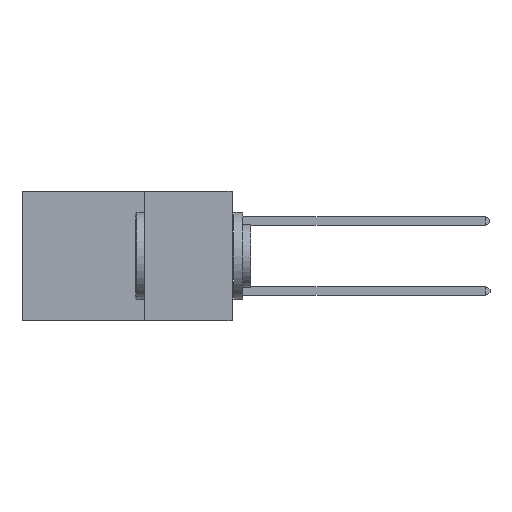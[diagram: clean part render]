
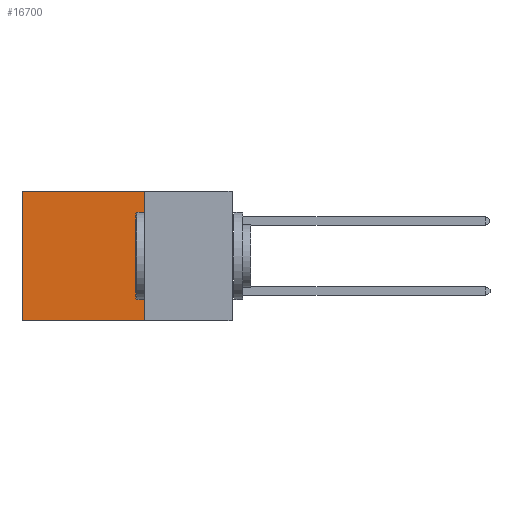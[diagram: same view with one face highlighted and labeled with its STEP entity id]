
A CAD part, left-side view. The second image highlights one B-rep face of the part: STEP entity #16700.
In plain terms, the highlighted planar face has unit normal (-1, 0, 0).
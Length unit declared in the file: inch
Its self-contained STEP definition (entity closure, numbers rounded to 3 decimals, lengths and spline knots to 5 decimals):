
#1242 = ORIENTED_EDGE ( 'NONE', *, *, #16120, .F. ) ;
#1254 = VECTOR ( 'NONE', #3936, 39.37008 ) ;
#3865 = VERTEX_POINT ( 'NONE', #8342 ) ;
#3936 = DIRECTION ( 'NONE',  ( 0., 0., -1. ) ) ;
#3940 = VERTEX_POINT ( 'NONE', #5247 ) ;
#5247 = CARTESIAN_POINT ( 'NONE',  ( 0.2875, 0.6, -0.37 ) ) ;
#5428 = LINE ( 'NONE', #10939, #1254 ) ;
#6461 = PLANE ( 'NONE',  #10349 ) ;
#6723 = CARTESIAN_POINT ( 'NONE',  ( 0.2875, 0.25, 0. ) ) ;
#7794 = EDGE_CURVE ( 'NONE', #13338, #8580, #21814, .T. ) ;
#8181 = DIRECTION ( 'NONE',  ( 0., 1., 0. ) ) ;
#8248 = DIRECTION ( 'NONE',  ( 0., 0., -1. ) ) ;
#8342 = CARTESIAN_POINT ( 'NONE',  ( 0.2875, 0.25, -0.37 ) ) ;
#8498 = DIRECTION ( 'NONE',  ( 0., 0., -1. ) ) ;
#8580 = VERTEX_POINT ( 'NONE', #8607 ) ;
#8607 = CARTESIAN_POINT ( 'NONE',  ( 0.2875, 0.6, 0. ) ) ;
#10349 = AXIS2_PLACEMENT_3D ( 'NONE', #11656, #18515, #8248 ) ;
#10939 = CARTESIAN_POINT ( 'NONE',  ( 0.2875, 0.6, 0. ) ) ;
#11174 = VECTOR ( 'NONE', #8181, 39.37008 ) ;
#11467 = ORIENTED_EDGE ( 'NONE', *, *, #13284, .T. ) ;
#11656 = CARTESIAN_POINT ( 'NONE',  ( 0.2875, 0.25, 0. ) ) ;
#12114 = VECTOR ( 'NONE', #22296, 39.37008 ) ;
#12118 = CARTESIAN_POINT ( 'NONE',  ( 0.2875, 0.25, -0.37 ) ) ;
#13183 = VECTOR ( 'NONE', #8498, 39.37008 ) ;
#13284 = EDGE_CURVE ( 'NONE', #8580, #3940, #5428, .T. ) ;
#13338 = VERTEX_POINT ( 'NONE', #19707 ) ;
#13375 = CARTESIAN_POINT ( 'NONE',  ( 0.2875, 0.25, 0. ) ) ;
#15078 = ORIENTED_EDGE ( 'NONE', *, *, #16183, .F. ) ;
#16120 = EDGE_CURVE ( 'NONE', #13338, #3865, #18810, .T. ) ;
#16183 = EDGE_CURVE ( 'NONE', #3865, #3940, #17768, .T. ) ;
#16700 = ADVANCED_FACE ( 'NONE', ( #21772 ), #6461, .F. ) ;
#17768 = LINE ( 'NONE', #12118, #12114 ) ;
#18515 = DIRECTION ( 'NONE',  ( 1., 0., 0. ) ) ;
#18810 = LINE ( 'NONE', #6723, #13183 ) ;
#19178 = EDGE_LOOP ( 'NONE', ( #11467, #15078, #1242, #19309 ) ) ;
#19309 = ORIENTED_EDGE ( 'NONE', *, *, #7794, .T. ) ;
#19707 = CARTESIAN_POINT ( 'NONE',  ( 0.2875, 0.25, 0. ) ) ;
#21772 = FACE_OUTER_BOUND ( 'NONE', #19178, .T. ) ;
#21814 = LINE ( 'NONE', #13375, #11174 ) ;
#22296 = DIRECTION ( 'NONE',  ( 0., 1., 0. ) ) ;
